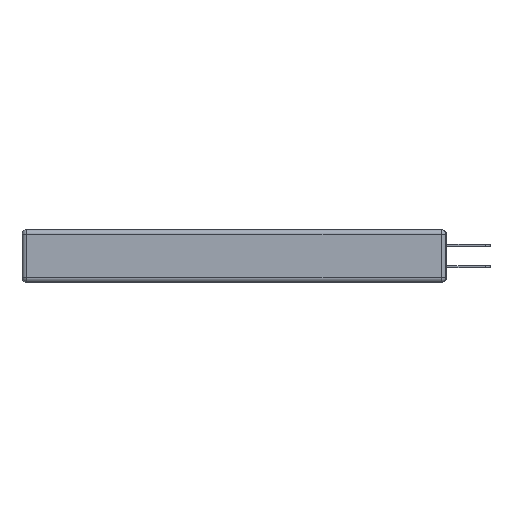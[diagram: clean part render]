
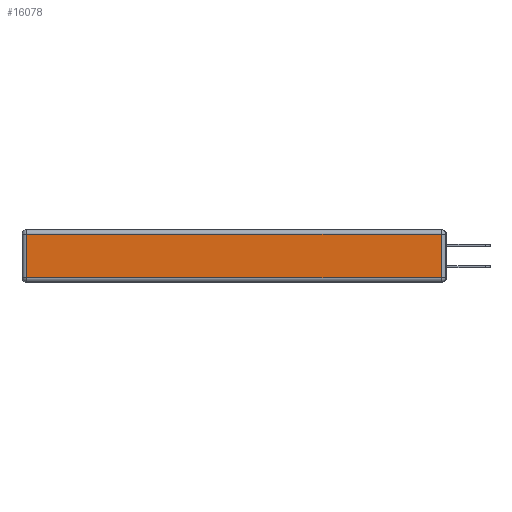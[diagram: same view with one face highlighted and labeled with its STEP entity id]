
A CAD part, left-side view. The second image highlights one B-rep face of the part: STEP entity #16078.
In plain terms, the highlighted planar face has unit normal (-1, 0, 0).
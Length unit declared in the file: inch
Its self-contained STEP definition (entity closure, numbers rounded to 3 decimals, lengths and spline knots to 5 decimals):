
#117 = CARTESIAN_POINT ( 'NONE',  ( 0., 2.72, -0.313 ) ) ;
#457 = LINE ( 'NONE', #7038, #6322 ) ;
#472 = LINE ( 'NONE', #4342, #2334 ) ;
#930 = DIRECTION ( 'NONE',  ( 0., -1., 0. ) ) ;
#1286 = VERTEX_POINT ( 'NONE', #13065 ) ;
#1671 = DIRECTION ( 'NONE',  ( 0., 1., 0. ) ) ;
#2334 = VECTOR ( 'NONE', #1671, 39.37008 ) ;
#2413 = AXIS2_PLACEMENT_3D ( 'NONE', #6531, #13240, #3932 ) ;
#2582 = PLANE ( 'NONE',  #2413 ) ;
#3221 = EDGE_CURVE ( 'NONE', #6511, #13193, #457, .T. ) ;
#3723 = CARTESIAN_POINT ( 'NONE',  ( 0., 0.03, -0.343 ) ) ;
#3932 = DIRECTION ( 'NONE',  ( 0., 0., 1. ) ) ;
#4342 = CARTESIAN_POINT ( 'NONE',  ( 0., 2.75, -0.03 ) ) ;
#4634 = VECTOR ( 'NONE', #930, 39.37008 ) ;
#4840 = ORIENTED_EDGE ( 'NONE', *, *, #3221, .T. ) ;
#5117 = VERTEX_POINT ( 'NONE', #8191 ) ;
#5265 = CARTESIAN_POINT ( 'NONE',  ( 0., 2.72, -0.03 ) ) ;
#6322 = VECTOR ( 'NONE', #16593, 39.37008 ) ;
#6511 = VERTEX_POINT ( 'NONE', #5265 ) ;
#6531 = CARTESIAN_POINT ( 'NONE',  ( 0., 0., -0.343 ) ) ;
#7038 = CARTESIAN_POINT ( 'NONE',  ( 0., 2.72, -0.343 ) ) ;
#7336 = ORIENTED_EDGE ( 'NONE', *, *, #8931, .T. ) ;
#8191 = CARTESIAN_POINT ( 'NONE',  ( 0., 0.03, -0.313 ) ) ;
#8226 = ORIENTED_EDGE ( 'NONE', *, *, #9141, .T. ) ;
#8240 = LINE ( 'NONE', #3723, #17179 ) ;
#8321 = ORIENTED_EDGE ( 'NONE', *, *, #15228, .T. ) ;
#8931 = EDGE_CURVE ( 'NONE', #5117, #1286, #8240, .T. ) ;
#9141 = EDGE_CURVE ( 'NONE', #1286, #6511, #472, .T. ) ;
#10169 = LINE ( 'NONE', #10422, #4634 ) ;
#10422 = CARTESIAN_POINT ( 'NONE',  ( 0., 0., -0.313 ) ) ;
#11229 = FACE_OUTER_BOUND ( 'NONE', #17324, .T. ) ;
#13065 = CARTESIAN_POINT ( 'NONE',  ( 0., 0.03, -0.03 ) ) ;
#13193 = VERTEX_POINT ( 'NONE', #117 ) ;
#13240 = DIRECTION ( 'NONE',  ( -1., 0., 0. ) ) ;
#15228 = EDGE_CURVE ( 'NONE', #13193, #5117, #10169, .T. ) ;
#16078 = ADVANCED_FACE ( 'NONE', ( #11229 ), #2582, .T. ) ;
#16593 = DIRECTION ( 'NONE',  ( 0., 0., -1. ) ) ;
#17179 = VECTOR ( 'NONE', #17361, 39.37008 ) ;
#17324 = EDGE_LOOP ( 'NONE', ( #8321, #7336, #8226, #4840 ) ) ;
#17361 = DIRECTION ( 'NONE',  ( 0., 0., 1. ) ) ;
